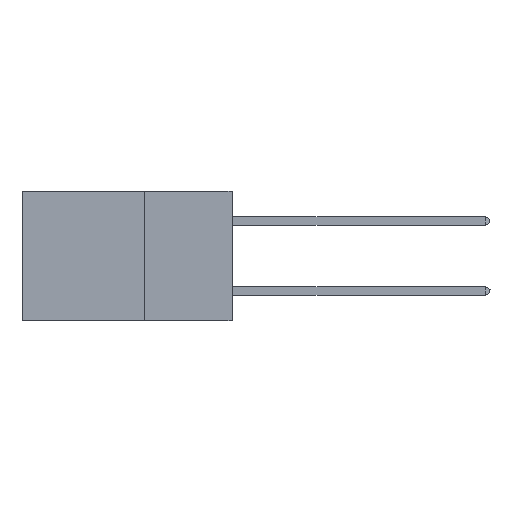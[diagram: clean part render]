
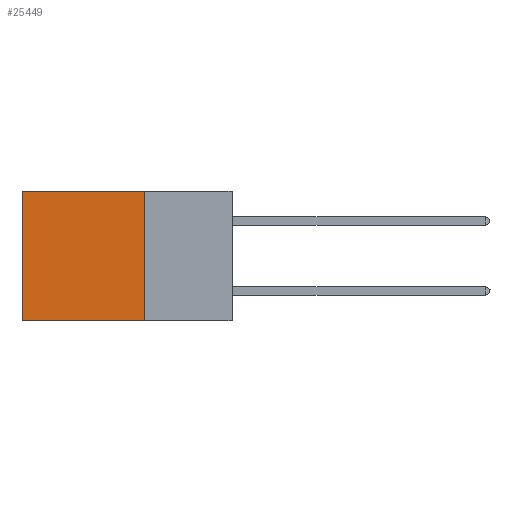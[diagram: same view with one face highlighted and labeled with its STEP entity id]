
A CAD part, left-side view. The second image highlights one B-rep face of the part: STEP entity #25449.
In plain terms, the highlighted planar face has unit normal (-1, 0, 0).
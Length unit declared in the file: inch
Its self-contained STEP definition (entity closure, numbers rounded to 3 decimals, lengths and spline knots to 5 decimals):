
#1672 = DIRECTION ( 'NONE',  ( 0., 0., -1. ) ) ;
#2136 = AXIS2_PLACEMENT_3D ( 'NONE', #7661, #28840, #14662 ) ;
#3292 = ORIENTED_EDGE ( 'NONE', *, *, #8906, .T. ) ;
#4391 = CARTESIAN_POINT ( 'NONE',  ( 0.2875, 0.25, 0. ) ) ;
#6195 = ORIENTED_EDGE ( 'NONE', *, *, #6281, .T. ) ;
#6223 = CARTESIAN_POINT ( 'NONE',  ( 0.2875, 0.25, -0.37 ) ) ;
#6281 = EDGE_CURVE ( 'NONE', #10338, #20687, #28685, .T. ) ;
#6549 = ORIENTED_EDGE ( 'NONE', *, *, #6926, .F. ) ;
#6685 = DIRECTION ( 'NONE',  ( 0., 1., 0. ) ) ;
#6926 = EDGE_CURVE ( 'NONE', #20703, #21116, #10567, .T. ) ;
#7661 = CARTESIAN_POINT ( 'NONE',  ( 0.2875, 0.25, 0. ) ) ;
#8667 = VECTOR ( 'NONE', #9273, 39.37008 ) ;
#8668 = CARTESIAN_POINT ( 'NONE',  ( 0.2875, 0.25, -0.37 ) ) ;
#8906 = EDGE_CURVE ( 'NONE', #20703, #10338, #11501, .T. ) ;
#9273 = DIRECTION ( 'NONE',  ( 0., 1., 0. ) ) ;
#9387 = CARTESIAN_POINT ( 'NONE',  ( 0.2875, 0.6, 0. ) ) ;
#10338 = VERTEX_POINT ( 'NONE', #21757 ) ;
#10567 = LINE ( 'NONE', #20982, #26730 ) ;
#11501 = LINE ( 'NONE', #15573, #14093 ) ;
#13174 = EDGE_LOOP ( 'NONE', ( #6195, #22306, #6549, #3292 ) ) ;
#14093 = VECTOR ( 'NONE', #6685, 39.37008 ) ;
#14662 = DIRECTION ( 'NONE',  ( 0., 0., -1. ) ) ;
#15138 = PLANE ( 'NONE',  #2136 ) ;
#15573 = CARTESIAN_POINT ( 'NONE',  ( 0.2875, 0.25, 0. ) ) ;
#19170 = DIRECTION ( 'NONE',  ( 0., 0., -1. ) ) ;
#19320 = FACE_OUTER_BOUND ( 'NONE', #13174, .T. ) ;
#19442 = VECTOR ( 'NONE', #19170, 39.37008 ) ;
#20687 = VERTEX_POINT ( 'NONE', #20890 ) ;
#20703 = VERTEX_POINT ( 'NONE', #4391 ) ;
#20890 = CARTESIAN_POINT ( 'NONE',  ( 0.2875, 0.6, -0.37 ) ) ;
#20982 = CARTESIAN_POINT ( 'NONE',  ( 0.2875, 0.25, 0. ) ) ;
#21116 = VERTEX_POINT ( 'NONE', #6223 ) ;
#21757 = CARTESIAN_POINT ( 'NONE',  ( 0.2875, 0.6, 0. ) ) ;
#22306 = ORIENTED_EDGE ( 'NONE', *, *, #26525, .F. ) ;
#25328 = LINE ( 'NONE', #8668, #8667 ) ;
#25449 = ADVANCED_FACE ( 'NONE', ( #19320 ), #15138, .F. ) ;
#26525 = EDGE_CURVE ( 'NONE', #21116, #20687, #25328, .T. ) ;
#26730 = VECTOR ( 'NONE', #1672, 39.37008 ) ;
#28685 = LINE ( 'NONE', #9387, #19442 ) ;
#28840 = DIRECTION ( 'NONE',  ( 1., 0., 0. ) ) ;
